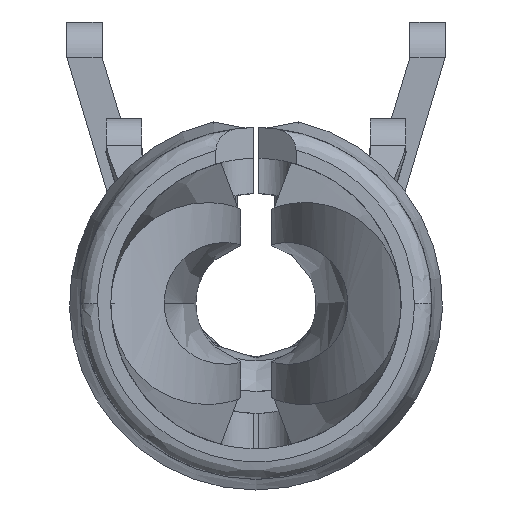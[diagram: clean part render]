
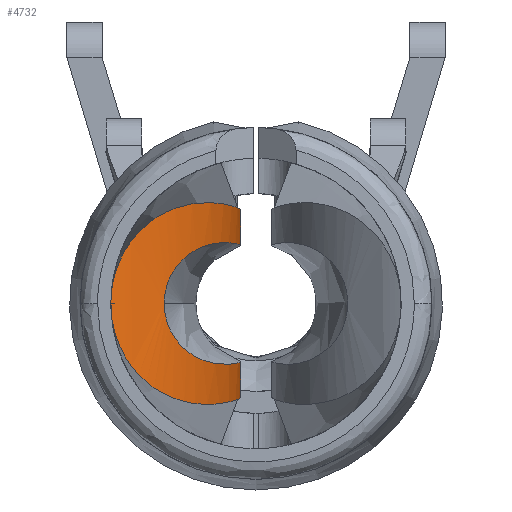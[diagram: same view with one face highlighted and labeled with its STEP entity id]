
A CAD part, front view. The second image highlights one B-rep face of the part: STEP entity #4732.
In plain terms, the highlighted cylindrical face has radius 1.517 mm (diameter 3.034 mm), a partial arc.
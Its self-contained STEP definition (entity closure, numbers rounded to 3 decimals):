
#38 = VECTOR ( 'NONE', #3786, 1000. ) ;
#64 = CARTESIAN_POINT ( 'NONE',  ( -0.087, -6.348, -0.33 ) ) ;
#72 = CARTESIAN_POINT ( 'NONE',  ( -0.111, -6.658, -0.55 ) ) ;
#88 = CARTESIAN_POINT ( 'NONE',  ( -0.087, -6.348, 0.33 ) ) ;
#234 = CARTESIAN_POINT ( 'NONE',  ( -0.205, -6.954, 0.571 ) ) ;
#282 = CYLINDRICAL_SURFACE ( 'NONE', #4822, 1.517 ) ;
#304 = CARTESIAN_POINT ( 'NONE',  ( -0.825, -7.65, 0. ) ) ;
#421 = ORIENTED_EDGE ( 'NONE', *, *, #5176, .T. ) ;
#470 = CARTESIAN_POINT ( 'NONE',  ( -0.507, -7.397, 0.112 ) ) ;
#536 = DIRECTION ( 'NONE',  ( 0., 0., 1. ) ) ;
#539 = CARTESIAN_POINT ( 'NONE',  ( -0.562, -7.454, -0.495 ) ) ;
#786 = B_SPLINE_CURVE_WITH_KNOTS ( 'NONE', 3,
 ( #2876, #1438, #2971, #4998, #2600, #6322, #539, #2134, #1599, #1075, #2526, #72, #1043, #4676 ),
 .UNSPECIFIED., .F., .F.,
 ( 4, 2, 2, 2, 2, 2, 4 ),
 ( 0.002, 0.002, 0.003, 0.003, 0.003, 0.003, 0.004 ),
 .UNSPECIFIED. ) ;
#868 = CARTESIAN_POINT ( 'NONE',  ( -0.148, -6.788, 0.346 ) ) ;
#958 = B_SPLINE_CURVE_WITH_KNOTS ( 'NONE', 3,
 ( #3011, #5037, #470, #3548, #2973, #3973, #6487, #2494, #868, #4542, #6555, #4944 ),
 .UNSPECIFIED., .F., .F.,
 ( 4, 2, 2, 2, 2, 4 ),
 ( 0.002, 0.002, 0.002, 0.002, 0.003, 0.003 ),
 .UNSPECIFIED. ) ;
#1043 = CARTESIAN_POINT ( 'NONE',  ( -0.087, -6.505, -0.538 ) ) ;
#1075 = CARTESIAN_POINT ( 'NONE',  ( -0.275, -7.096, -0.581 ) ) ;
#1400 = CARTESIAN_POINT ( 'NONE',  ( -0.507, -7.397, -0.112 ) ) ;
#1438 = CARTESIAN_POINT ( 'NONE',  ( -0.825, -7.65, -0.079 ) ) ;
#1479 = ORIENTED_EDGE ( 'NONE', *, *, #2294, .T. ) ;
#1599 = CARTESIAN_POINT ( 'NONE',  ( -0.41, -7.287, -0.559 ) ) ;
#1636 = ORIENTED_EDGE ( 'NONE', *, *, #2648, .T. ) ;
#1829 = CARTESIAN_POINT ( 'NONE',  ( -0.184, -6.894, -0.349 ) ) ;
#2134 = CARTESIAN_POINT ( 'NONE',  ( -0.459, -7.346, -0.545 ) ) ;
#2243 = CARTESIAN_POINT ( 'NONE',  ( -0.148, -6.789, -0.346 ) ) ;
#2294 = EDGE_CURVE ( 'NONE', #2738, #4078, #2781, .T. ) ;
#2307 = DIRECTION ( 'NONE',  ( 0., 0., 1. ) ) ;
#2325 = CARTESIAN_POINT ( 'NONE',  ( -0.087, -6.503, 0.538 ) ) ;
#2338 = CARTESIAN_POINT ( 'NONE',  ( -1.604, -6.348, 0. ) ) ;
#2354 = EDGE_CURVE ( 'NONE', #6391, #4619, #958, .T. ) ;
#2494 = CARTESIAN_POINT ( 'NONE',  ( -0.184, -6.895, 0.349 ) ) ;
#2526 = CARTESIAN_POINT ( 'NONE',  ( -0.205, -6.956, -0.571 ) ) ;
#2600 = CARTESIAN_POINT ( 'NONE',  ( -0.711, -7.576, -0.36 ) ) ;
#2648 = EDGE_CURVE ( 'NONE', #4619, #4583, #4607, .T. ) ;
#2738 = VERTEX_POINT ( 'NONE', #5305 ) ;
#2752 = CARTESIAN_POINT ( 'NONE',  ( -0.087, -6.348, -0.33 ) ) ;
#2756 = ORIENTED_EDGE ( 'NONE', *, *, #4519, .T. ) ;
#2761 = EDGE_LOOP ( 'NONE', ( #4912, #421, #1479, #2756, #2780, #1636 ) ) ;
#2780 = ORIENTED_EDGE ( 'NONE', *, *, #2354, .T. ) ;
#2781 = LINE ( 'NONE', #3256, #38 ) ;
#2876 = CARTESIAN_POINT ( 'NONE',  ( -0.825, -7.65, 0. ) ) ;
#2905 = CARTESIAN_POINT ( 'NONE',  ( -0.275, -7.096, 0.581 ) ) ;
#2971 = CARTESIAN_POINT ( 'NONE',  ( -0.809, -7.641, -0.157 ) ) ;
#2973 = CARTESIAN_POINT ( 'NONE',  ( -0.431, -7.312, 0.237 ) ) ;
#3011 = CARTESIAN_POINT ( 'NONE',  ( -0.522, -7.411, 0. ) ) ;
#3012 = CARTESIAN_POINT ( 'NONE',  ( -0.522, -7.411, 0. ) ) ;
#3075 = CARTESIAN_POINT ( 'NONE',  ( -0.087, -6.348, 0. ) ) ;
#3256 = CARTESIAN_POINT ( 'NONE',  ( -0.087, -6.348, 0. ) ) ;
#3280 = CARTESIAN_POINT ( 'NONE',  ( -0.562, -7.453, 0.495 ) ) ;
#3332 = B_SPLINE_CURVE_WITH_KNOTS ( 'NONE', 3,
 ( #2752, #4788, #6307, #2243, #1829, #3757, #3909, #5778, #5256, #1400, #5402, #3938 ),
 .UNSPECIFIED., .F., .F.,
 ( 4, 2, 2, 2, 2, 4 ),
 ( 0., 0.001, 0.001, 0.001, 0.001, 0.002 ),
 .UNSPECIFIED. ) ;
#3548 = CARTESIAN_POINT ( 'NONE',  ( -0.461, -7.347, 0.202 ) ) ;
#3757 = CARTESIAN_POINT ( 'NONE',  ( -0.28, -7.097, -0.334 ) ) ;
#3780 = CARTESIAN_POINT ( 'NONE',  ( -0.111, -6.659, 0.55 ) ) ;
#3786 = DIRECTION ( 'NONE',  ( 0., 0., 1. ) ) ;
#3791 = FACE_OUTER_BOUND ( 'NONE', #2761, .T. ) ;
#3842 = CARTESIAN_POINT ( 'NONE',  ( -0.459, -7.346, 0.545 ) ) ;
#3909 = CARTESIAN_POINT ( 'NONE',  ( -0.341, -7.194, -0.315 ) ) ;
#3938 = CARTESIAN_POINT ( 'NONE',  ( -0.522, -7.411, 0. ) ) ;
#3973 = CARTESIAN_POINT ( 'NONE',  ( -0.34, -7.193, 0.316 ) ) ;
#4071 = CARTESIAN_POINT ( 'NONE',  ( -0.825, -7.65, 0. ) ) ;
#4078 = VERTEX_POINT ( 'NONE', #64 ) ;
#4273 = CARTESIAN_POINT ( 'NONE',  ( -0.809, -7.641, 0.157 ) ) ;
#4365 = CARTESIAN_POINT ( 'NONE',  ( -0.409, -7.286, 0.559 ) ) ;
#4381 = DIRECTION ( 'NONE',  ( 1., 0., 0. ) ) ;
#4409 = VECTOR ( 'NONE', #536, 1000. ) ;
#4449 = B_SPLINE_CURVE_WITH_KNOTS ( 'NONE', 3,
 ( #5306, #2325, #3780, #234, #2905, #4365, #3842, #3280, #5427, #6328, #6390, #4273, #5797, #304 ),
 .UNSPECIFIED., .F., .F.,
 ( 4, 2, 2, 2, 2, 2, 4 ),
 ( 0., 0.001, 0.001, 0.001, 0.002, 0.002, 0.002 ),
 .UNSPECIFIED. ) ;
#4519 = EDGE_CURVE ( 'NONE', #4078, #6391, #3332, .T. ) ;
#4542 = CARTESIAN_POINT ( 'NONE',  ( -0.099, -6.57, 0.338 ) ) ;
#4583 = VERTEX_POINT ( 'NONE', #6020 ) ;
#4607 = LINE ( 'NONE', #3075, #4409 ) ;
#4619 = VERTEX_POINT ( 'NONE', #88 ) ;
#4676 = CARTESIAN_POINT ( 'NONE',  ( -0.087, -6.348, -0.534 ) ) ;
#4732 = ADVANCED_FACE ( 'NONE', ( #3791 ), #282, .T. ) ;
#4788 = CARTESIAN_POINT ( 'NONE',  ( -0.087, -6.459, -0.332 ) ) ;
#4822 = AXIS2_PLACEMENT_3D ( 'NONE', #2338, #2307, #4381 ) ;
#4912 = ORIENTED_EDGE ( 'NONE', *, *, #6544, .T. ) ;
#4944 = CARTESIAN_POINT ( 'NONE',  ( -0.087, -6.348, 0.33 ) ) ;
#4998 = CARTESIAN_POINT ( 'NONE',  ( -0.753, -7.604, -0.298 ) ) ;
#5037 = CARTESIAN_POINT ( 'NONE',  ( -0.522, -7.411, 0.056 ) ) ;
#5176 = EDGE_CURVE ( 'NONE', #5792, #2738, #786, .T. ) ;
#5256 = CARTESIAN_POINT ( 'NONE',  ( -0.461, -7.347, -0.203 ) ) ;
#5305 = CARTESIAN_POINT ( 'NONE',  ( -0.087, -6.348, -0.534 ) ) ;
#5306 = CARTESIAN_POINT ( 'NONE',  ( -0.087, -6.348, 0.534 ) ) ;
#5402 = CARTESIAN_POINT ( 'NONE',  ( -0.522, -7.411, -0.056 ) ) ;
#5427 = CARTESIAN_POINT ( 'NONE',  ( -0.615, -7.5, 0.459 ) ) ;
#5778 = CARTESIAN_POINT ( 'NONE',  ( -0.431, -7.312, -0.238 ) ) ;
#5792 = VERTEX_POINT ( 'NONE', #4071 ) ;
#5797 = CARTESIAN_POINT ( 'NONE',  ( -0.825, -7.65, 0.079 ) ) ;
#6020 = CARTESIAN_POINT ( 'NONE',  ( -0.087, -6.348, 0.534 ) ) ;
#6307 = CARTESIAN_POINT ( 'NONE',  ( -0.099, -6.57, -0.338 ) ) ;
#6322 = CARTESIAN_POINT ( 'NONE',  ( -0.615, -7.501, -0.459 ) ) ;
#6328 = CARTESIAN_POINT ( 'NONE',  ( -0.71, -7.576, 0.361 ) ) ;
#6390 = CARTESIAN_POINT ( 'NONE',  ( -0.752, -7.604, 0.298 ) ) ;
#6391 = VERTEX_POINT ( 'NONE', #3012 ) ;
#6487 = CARTESIAN_POINT ( 'NONE',  ( -0.279, -7.096, 0.334 ) ) ;
#6544 = EDGE_CURVE ( 'NONE', #4583, #5792, #4449, .T. ) ;
#6555 = CARTESIAN_POINT ( 'NONE',  ( -0.087, -6.46, 0.332 ) ) ;
